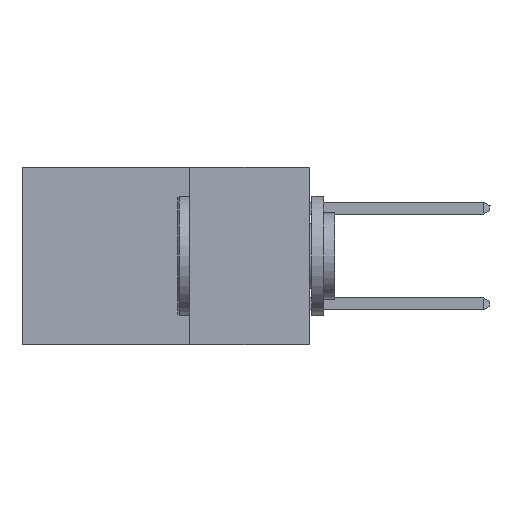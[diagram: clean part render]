
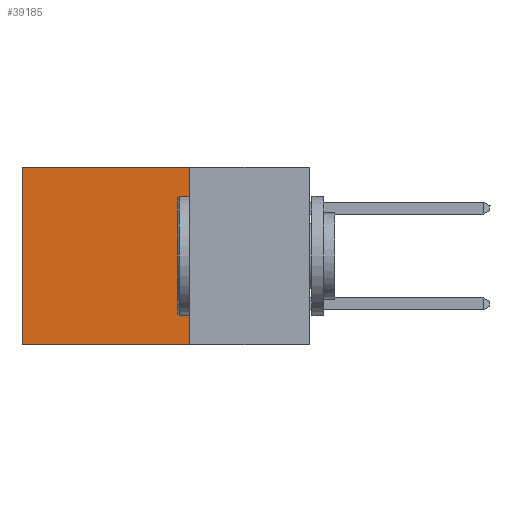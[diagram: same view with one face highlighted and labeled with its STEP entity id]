
A CAD part, left-side view. The second image highlights one B-rep face of the part: STEP entity #39185.
In plain terms, the highlighted planar face has unit normal (-1, 0, 0).
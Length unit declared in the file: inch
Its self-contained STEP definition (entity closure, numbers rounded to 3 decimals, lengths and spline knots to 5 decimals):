
#77 = DIRECTION ( 'NONE',  ( 0., 0., -1. ) ) ;
#344 = DIRECTION ( 'NONE',  ( 0., 1., 0. ) ) ;
#579 = VECTOR ( 'NONE', #21929, 39.37008 ) ;
#1331 = VECTOR ( 'NONE', #10121, 39.37008 ) ;
#2375 = LINE ( 'NONE', #13525, #1331 ) ;
#6420 = EDGE_CURVE ( 'NONE', #11388, #37670, #22313, .T. ) ;
#7441 = CARTESIAN_POINT ( 'NONE',  ( 0.2875, 0.6, -0.37 ) ) ;
#7688 = ORIENTED_EDGE ( 'NONE', *, *, #36585, .F. ) ;
#9514 = LINE ( 'NONE', #32056, #579 ) ;
#10121 = DIRECTION ( 'NONE',  ( 0., 1., 0. ) ) ;
#10562 = EDGE_CURVE ( 'NONE', #17583, #37670, #42357, .T. ) ;
#10903 = PLANE ( 'NONE',  #37554 ) ;
#11388 = VERTEX_POINT ( 'NONE', #40781 ) ;
#12192 = CARTESIAN_POINT ( 'NONE',  ( 0.2875, 0.25, 0. ) ) ;
#13525 = CARTESIAN_POINT ( 'NONE',  ( 0.2875, 0.25, 0. ) ) ;
#15517 = ORIENTED_EDGE ( 'NONE', *, *, #20433, .T. ) ;
#15729 = VECTOR ( 'NONE', #77, 39.37008 ) ;
#17583 = VERTEX_POINT ( 'NONE', #31206 ) ;
#17663 = DIRECTION ( 'NONE',  ( 1., 0., 0. ) ) ;
#20433 = EDGE_CURVE ( 'NONE', #20929, #17583, #2375, .T. ) ;
#20508 = CARTESIAN_POINT ( 'NONE',  ( 0.2875, 0.25, -0.37 ) ) ;
#20929 = VERTEX_POINT ( 'NONE', #12192 ) ;
#21929 = DIRECTION ( 'NONE',  ( 0., 0., -1. ) ) ;
#22313 = LINE ( 'NONE', #20508, #41124 ) ;
#27609 = CARTESIAN_POINT ( 'NONE',  ( 0.2875, 0.25, 0. ) ) ;
#31206 = CARTESIAN_POINT ( 'NONE',  ( 0.2875, 0.6, 0. ) ) ;
#32056 = CARTESIAN_POINT ( 'NONE',  ( 0.2875, 0.25, 0. ) ) ;
#32883 = EDGE_LOOP ( 'NONE', ( #39226, #36377, #7688, #15517 ) ) ;
#36377 = ORIENTED_EDGE ( 'NONE', *, *, #6420, .F. ) ;
#36585 = EDGE_CURVE ( 'NONE', #20929, #11388, #9514, .T. ) ;
#37554 = AXIS2_PLACEMENT_3D ( 'NONE', #27609, #17663, #41031 ) ;
#37670 = VERTEX_POINT ( 'NONE', #7441 ) ;
#39185 = ADVANCED_FACE ( 'NONE', ( #41470 ), #10903, .F. ) ;
#39226 = ORIENTED_EDGE ( 'NONE', *, *, #10562, .T. ) ;
#40252 = CARTESIAN_POINT ( 'NONE',  ( 0.2875, 0.6, 0. ) ) ;
#40781 = CARTESIAN_POINT ( 'NONE',  ( 0.2875, 0.25, -0.37 ) ) ;
#41031 = DIRECTION ( 'NONE',  ( 0., 0., -1. ) ) ;
#41124 = VECTOR ( 'NONE', #344, 39.37008 ) ;
#41470 = FACE_OUTER_BOUND ( 'NONE', #32883, .T. ) ;
#42357 = LINE ( 'NONE', #40252, #15729 ) ;
